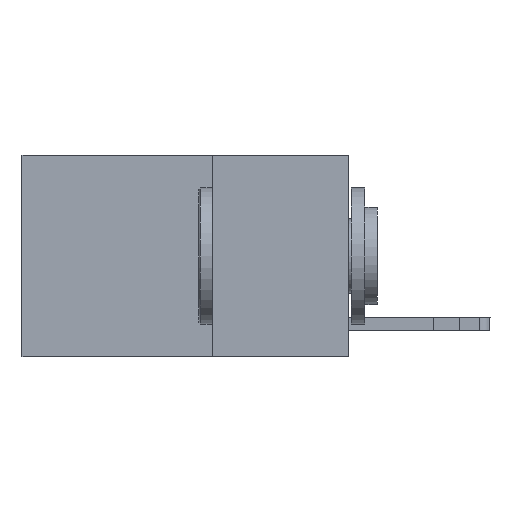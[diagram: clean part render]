
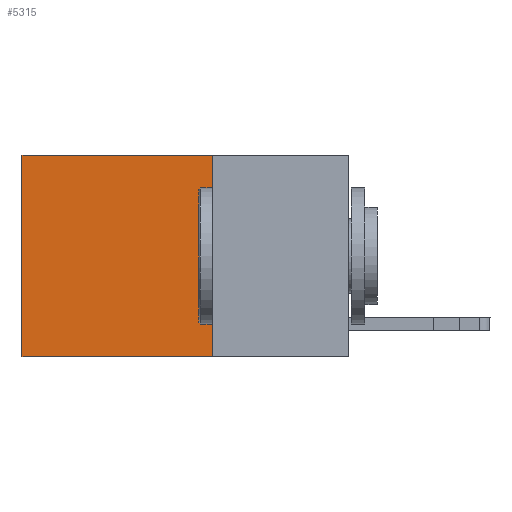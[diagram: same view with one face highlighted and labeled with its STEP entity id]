
A CAD part, left-side view. The second image highlights one B-rep face of the part: STEP entity #5315.
In plain terms, the highlighted planar face has unit normal (-1, 0, 0).
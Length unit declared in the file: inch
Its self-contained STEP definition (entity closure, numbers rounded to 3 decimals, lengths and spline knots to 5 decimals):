
#1713 = EDGE_CURVE ( 'NONE', #2244, #17699, #17196, .T. ) ;
#2244 = VERTEX_POINT ( 'NONE', #6780 ) ;
#3076 = ORIENTED_EDGE ( 'NONE', *, *, #8121, .T. ) ;
#3083 = DIRECTION ( 'NONE',  ( 0., 0., -1. ) ) ;
#3653 = VERTEX_POINT ( 'NONE', #15130 ) ;
#5315 = ADVANCED_FACE ( 'NONE', ( #19847 ), #5753, .F. ) ;
#5753 = PLANE ( 'NONE',  #12495 ) ;
#6056 = CARTESIAN_POINT ( 'NONE',  ( 0.2625, 0.25, -0.37 ) ) ;
#6639 = ORIENTED_EDGE ( 'NONE', *, *, #9484, .F. ) ;
#6780 = CARTESIAN_POINT ( 'NONE',  ( 0.2625, 0.25, 0. ) ) ;
#7577 = LINE ( 'NONE', #18877, #19815 ) ;
#8121 = EDGE_CURVE ( 'NONE', #17699, #3653, #7577, .T. ) ;
#9484 = EDGE_CURVE ( 'NONE', #2244, #19976, #15709, .T. ) ;
#10815 = DIRECTION ( 'NONE',  ( 0., 1., 0. ) ) ;
#10921 = VECTOR ( 'NONE', #3083, 39.37008 ) ;
#11156 = CARTESIAN_POINT ( 'NONE',  ( 0.2625, 0.25, -0.37 ) ) ;
#12041 = CARTESIAN_POINT ( 'NONE',  ( 0.2625, 0.25, 0. ) ) ;
#12495 = AXIS2_PLACEMENT_3D ( 'NONE', #12041, #13669, #19944 ) ;
#12752 = ORIENTED_EDGE ( 'NONE', *, *, #14141, .F. ) ;
#13669 = DIRECTION ( 'NONE',  ( 1., 0., 0. ) ) ;
#14141 = EDGE_CURVE ( 'NONE', #19976, #3653, #16866, .T. ) ;
#15130 = CARTESIAN_POINT ( 'NONE',  ( 0.2625, 0.6, -0.37 ) ) ;
#15316 = DIRECTION ( 'NONE',  ( 0., 1., 0. ) ) ;
#15709 = LINE ( 'NONE', #17060, #10921 ) ;
#16253 = VECTOR ( 'NONE', #15316, 39.37008 ) ;
#16302 = ORIENTED_EDGE ( 'NONE', *, *, #1713, .T. ) ;
#16866 = LINE ( 'NONE', #6056, #16253 ) ;
#16993 = VECTOR ( 'NONE', #10815, 39.37008 ) ;
#17060 = CARTESIAN_POINT ( 'NONE',  ( 0.2625, 0.25, 0. ) ) ;
#17196 = LINE ( 'NONE', #20272, #16993 ) ;
#17536 = DIRECTION ( 'NONE',  ( 0., 0., -1. ) ) ;
#17699 = VERTEX_POINT ( 'NONE', #18952 ) ;
#18877 = CARTESIAN_POINT ( 'NONE',  ( 0.2625, 0.6, 0. ) ) ;
#18952 = CARTESIAN_POINT ( 'NONE',  ( 0.2625, 0.6, 0. ) ) ;
#19314 = EDGE_LOOP ( 'NONE', ( #3076, #12752, #6639, #16302 ) ) ;
#19815 = VECTOR ( 'NONE', #17536, 39.37008 ) ;
#19847 = FACE_OUTER_BOUND ( 'NONE', #19314, .T. ) ;
#19944 = DIRECTION ( 'NONE',  ( 0., 0., -1. ) ) ;
#19976 = VERTEX_POINT ( 'NONE', #11156 ) ;
#20272 = CARTESIAN_POINT ( 'NONE',  ( 0.2625, 0.25, 0. ) ) ;
